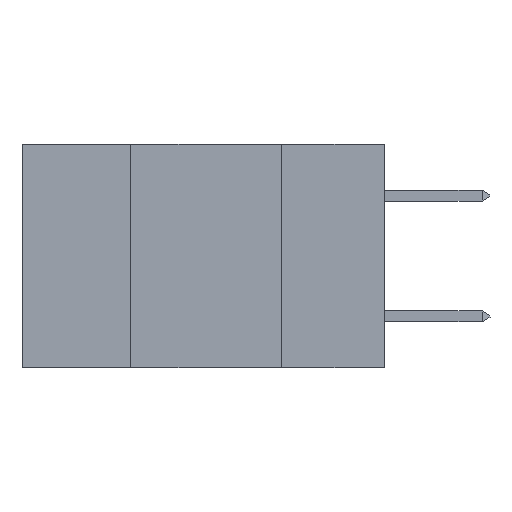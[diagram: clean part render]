
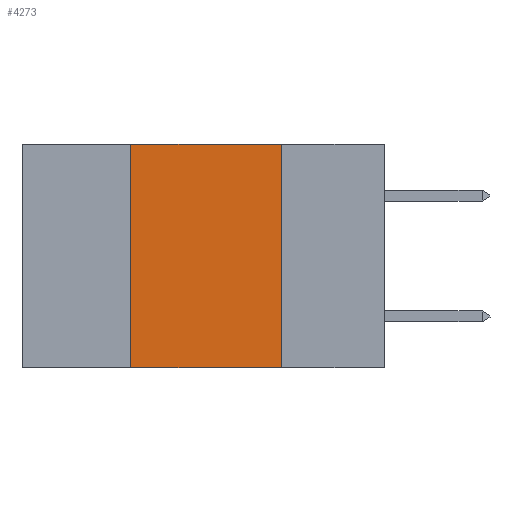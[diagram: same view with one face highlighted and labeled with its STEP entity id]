
A CAD part, left-side view. The second image highlights one B-rep face of the part: STEP entity #4273.
In plain terms, the highlighted planar face has unit normal (-1, 0, 0).
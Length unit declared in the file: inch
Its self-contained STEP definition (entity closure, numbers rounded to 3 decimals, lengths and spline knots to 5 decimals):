
#828 = CARTESIAN_POINT ( 'NONE',  ( 0., 0.42, 0. ) ) ;
#1373 = DIRECTION ( 'NONE',  ( 1., 0., 0. ) ) ;
#2154 = VECTOR ( 'NONE', #3420, 39.37008 ) ;
#2283 = DIRECTION ( 'NONE',  ( 0., 0., -1. ) ) ;
#2387 = LINE ( 'NONE', #5225, #4087 ) ;
#2480 = VERTEX_POINT ( 'NONE', #10277 ) ;
#2638 = EDGE_CURVE ( 'NONE', #3078, #2480, #3145, .T. ) ;
#2770 = ORIENTED_EDGE ( 'NONE', *, *, #3372, .T. ) ;
#3078 = VERTEX_POINT ( 'NONE', #828 ) ;
#3145 = LINE ( 'NONE', #3535, #2154 ) ;
#3372 = EDGE_CURVE ( 'NONE', #4830, #11077, #10865, .T. ) ;
#3420 = DIRECTION ( 'NONE',  ( 0., -1., 0. ) ) ;
#3535 = CARTESIAN_POINT ( 'NONE',  ( 0., 0.6, 0. ) ) ;
#4087 = VECTOR ( 'NONE', #9546, 39.37008 ) ;
#4187 = PLANE ( 'NONE',  #6848 ) ;
#4273 = ADVANCED_FACE ( 'NONE', ( #8163 ), #4187, .F. ) ;
#4830 = VERTEX_POINT ( 'NONE', #6987 ) ;
#4833 = DIRECTION ( 'NONE',  ( 0., -1., 0. ) ) ;
#4853 = EDGE_LOOP ( 'NONE', ( #9592, #10979, #5877, #2770 ) ) ;
#5225 = CARTESIAN_POINT ( 'NONE',  ( 0., 0.17, 0. ) ) ;
#5877 = ORIENTED_EDGE ( 'NONE', *, *, #8979, .F. ) ;
#5911 = CARTESIAN_POINT ( 'NONE',  ( 0., 0.6, 0. ) ) ;
#6029 = EDGE_CURVE ( 'NONE', #2480, #11077, #2387, .T. ) ;
#6574 = CARTESIAN_POINT ( 'NONE',  ( 0., 0.6, -0.37 ) ) ;
#6848 = AXIS2_PLACEMENT_3D ( 'NONE', #5911, #1373, #2283 ) ;
#6987 = CARTESIAN_POINT ( 'NONE',  ( 0., 0.42, -0.37 ) ) ;
#7426 = CARTESIAN_POINT ( 'NONE',  ( 0., 0.42, 0. ) ) ;
#7734 = DIRECTION ( 'NONE',  ( 0., 0., 1. ) ) ;
#8159 = VECTOR ( 'NONE', #4833, 39.37008 ) ;
#8163 = FACE_OUTER_BOUND ( 'NONE', #4853, .T. ) ;
#8979 = EDGE_CURVE ( 'NONE', #4830, #3078, #10451, .T. ) ;
#9059 = CARTESIAN_POINT ( 'NONE',  ( 0., 0.17, -0.37 ) ) ;
#9546 = DIRECTION ( 'NONE',  ( 0., 0., -1. ) ) ;
#9592 = ORIENTED_EDGE ( 'NONE', *, *, #6029, .F. ) ;
#10277 = CARTESIAN_POINT ( 'NONE',  ( 0., 0.17, 0. ) ) ;
#10451 = LINE ( 'NONE', #7426, #10746 ) ;
#10746 = VECTOR ( 'NONE', #7734, 39.37008 ) ;
#10865 = LINE ( 'NONE', #6574, #8159 ) ;
#10979 = ORIENTED_EDGE ( 'NONE', *, *, #2638, .F. ) ;
#11077 = VERTEX_POINT ( 'NONE', #9059 ) ;
